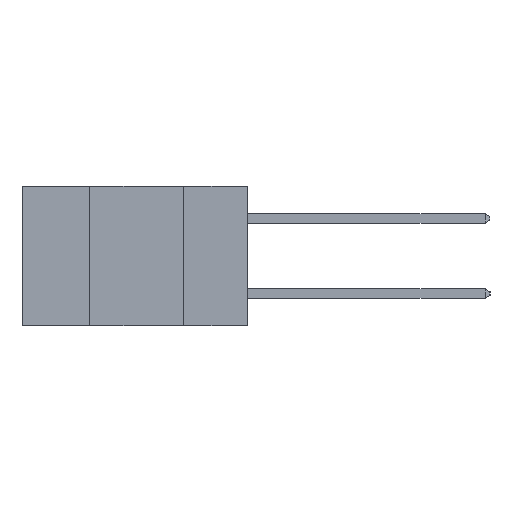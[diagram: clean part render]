
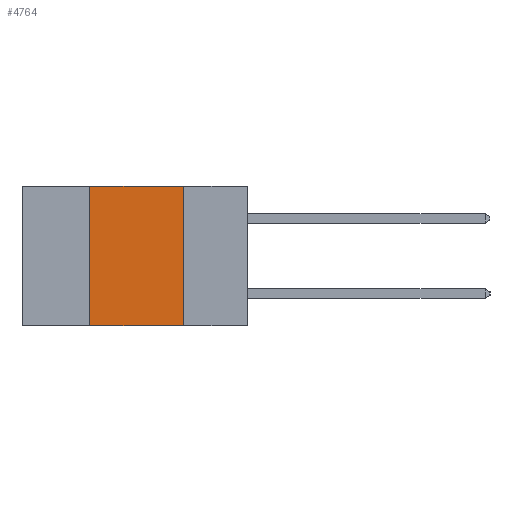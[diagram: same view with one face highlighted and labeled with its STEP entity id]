
A CAD part, left-side view. The second image highlights one B-rep face of the part: STEP entity #4764.
In plain terms, the highlighted planar face has unit normal (-1, 0, 0).
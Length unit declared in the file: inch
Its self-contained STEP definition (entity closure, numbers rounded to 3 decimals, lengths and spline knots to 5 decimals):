
#108 = EDGE_CURVE ( 'NONE', #12370, #8101, #2346, .T. ) ;
#420 = ORIENTED_EDGE ( 'NONE', *, *, #14507, .T. ) ;
#532 = VECTOR ( 'NONE', #7835, 39.37008 ) ;
#687 = DIRECTION ( 'NONE',  ( 1., 0., 0. ) ) ;
#843 = CARTESIAN_POINT ( 'NONE',  ( 0., 0.6, 0. ) ) ;
#1209 = ORIENTED_EDGE ( 'NONE', *, *, #2477, .F. ) ;
#2346 = LINE ( 'NONE', #10785, #2725 ) ;
#2477 = EDGE_CURVE ( 'NONE', #7077, #2506, #14710, .T. ) ;
#2506 = VERTEX_POINT ( 'NONE', #10800 ) ;
#2688 = PLANE ( 'NONE',  #12690 ) ;
#2725 = VECTOR ( 'NONE', #7820, 39.37008 ) ;
#3379 = CARTESIAN_POINT ( 'NONE',  ( 0., 0.42, 0. ) ) ;
#3824 = DIRECTION ( 'NONE',  ( 0., 0., -1. ) ) ;
#3842 = CARTESIAN_POINT ( 'NONE',  ( 0., 0.6, 0. ) ) ;
#4059 = EDGE_CURVE ( 'NONE', #8101, #7077, #12651, .T. ) ;
#4069 = ORIENTED_EDGE ( 'NONE', *, *, #4059, .F. ) ;
#4303 = DIRECTION ( 'NONE',  ( 0., 0., -1. ) ) ;
#4496 = CARTESIAN_POINT ( 'NONE',  ( 0., 0.17, -0.37 ) ) ;
#4764 = ADVANCED_FACE ( 'NONE', ( #7325 ), #2688, .F. ) ;
#5835 = VECTOR ( 'NONE', #4303, 39.37008 ) ;
#5921 = CARTESIAN_POINT ( 'NONE',  ( 0., 0.42, -0.37 ) ) ;
#7077 = VERTEX_POINT ( 'NONE', #9822 ) ;
#7325 = FACE_OUTER_BOUND ( 'NONE', #11721, .T. ) ;
#7820 = DIRECTION ( 'NONE',  ( 0., 0., 1. ) ) ;
#7835 = DIRECTION ( 'NONE',  ( 0., -1., 0. ) ) ;
#7852 = CARTESIAN_POINT ( 'NONE',  ( 0., 0.6, -0.37 ) ) ;
#8101 = VERTEX_POINT ( 'NONE', #3379 ) ;
#8930 = DIRECTION ( 'NONE',  ( 0., -1., 0. ) ) ;
#9822 = CARTESIAN_POINT ( 'NONE',  ( 0., 0.17, 0. ) ) ;
#10785 = CARTESIAN_POINT ( 'NONE',  ( 0., 0.42, -0.37 ) ) ;
#10800 = CARTESIAN_POINT ( 'NONE',  ( 0., 0.17, -0.37 ) ) ;
#11721 = EDGE_LOOP ( 'NONE', ( #1209, #4069, #13637, #420 ) ) ;
#12229 = LINE ( 'NONE', #7852, #532 ) ;
#12255 = VECTOR ( 'NONE', #8930, 39.37008 ) ;
#12370 = VERTEX_POINT ( 'NONE', #5921 ) ;
#12651 = LINE ( 'NONE', #843, #12255 ) ;
#12690 = AXIS2_PLACEMENT_3D ( 'NONE', #3842, #687, #3824 ) ;
#13637 = ORIENTED_EDGE ( 'NONE', *, *, #108, .F. ) ;
#14507 = EDGE_CURVE ( 'NONE', #12370, #2506, #12229, .T. ) ;
#14710 = LINE ( 'NONE', #4496, #5835 ) ;
